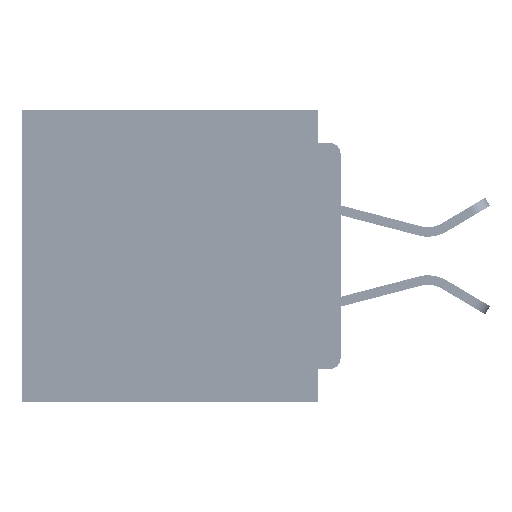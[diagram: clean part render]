
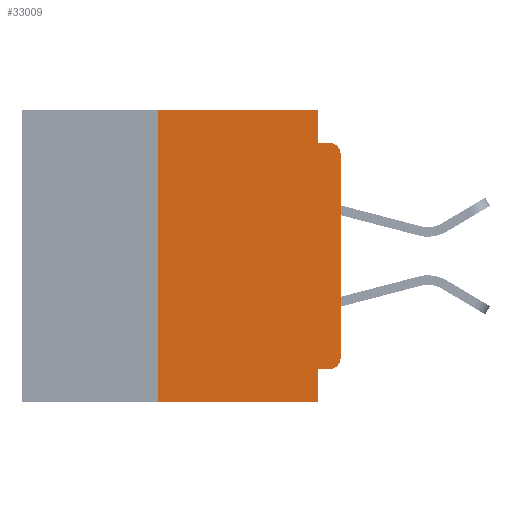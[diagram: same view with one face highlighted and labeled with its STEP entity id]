
A CAD part, left-side view. The second image highlights one B-rep face of the part: STEP entity #33009.
In plain terms, the highlighted planar face has unit normal (-1, 0, 0).
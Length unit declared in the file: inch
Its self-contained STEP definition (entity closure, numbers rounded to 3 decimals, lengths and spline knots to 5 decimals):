
#761 = CARTESIAN_POINT ( 'NONE',  ( 0., 0.031, -0.4 ) ) ;
#1078 = ORIENTED_EDGE ( 'NONE', *, *, #26324, .T. ) ;
#2343 = VECTOR ( 'NONE', #21626, 39.37008 ) ;
#2947 = AXIS2_PLACEMENT_3D ( 'NONE', #13943, #51163, #19364 ) ;
#2953 = DIRECTION ( 'NONE',  ( 0., 0., -1. ) ) ;
#3020 = VERTEX_POINT ( 'NONE', #41091 ) ;
#3185 = LINE ( 'NONE', #68620, #14150 ) ;
#3899 = VERTEX_POINT ( 'NONE', #10021 ) ;
#4468 = DIRECTION ( 'NONE',  ( 0., 0., 1. ) ) ;
#6984 = ORIENTED_EDGE ( 'NONE', *, *, #51844, .T. ) ;
#7105 = DIRECTION ( 'NONE',  ( 0., -1., 0. ) ) ;
#7507 = CARTESIAN_POINT ( 'NONE',  ( 0., 0.031, 0. ) ) ;
#8432 = CARTESIAN_POINT ( 'NONE',  ( 0., 0.437, -0.4 ) ) ;
#9477 = LINE ( 'NONE', #51518, #34702 ) ;
#10021 = CARTESIAN_POINT ( 'NONE',  ( 0., 0.015, -0.045 ) ) ;
#10410 = CIRCLE ( 'NONE', #2947, 0.015 ) ;
#11885 = CARTESIAN_POINT ( 'NONE',  ( 0., 0., -0.34 ) ) ;
#12005 = ORIENTED_EDGE ( 'NONE', *, *, #28152, .T. ) ;
#12892 = ORIENTED_EDGE ( 'NONE', *, *, #33095, .F. ) ;
#13035 = CARTESIAN_POINT ( 'NONE',  ( 0., 0.015, -0.34 ) ) ;
#13685 = VERTEX_POINT ( 'NONE', #55455 ) ;
#13847 = DIRECTION ( 'NONE',  ( 0., -1., 0. ) ) ;
#13943 = CARTESIAN_POINT ( 'NONE',  ( 0., 0.015, -0.06 ) ) ;
#14150 = VECTOR ( 'NONE', #31855, 39.37008 ) ;
#14158 = CARTESIAN_POINT ( 'NONE',  ( 0., 0.25, -0.4 ) ) ;
#15437 = VERTEX_POINT ( 'NONE', #17422 ) ;
#15997 = CARTESIAN_POINT ( 'NONE',  ( 0., 0.437, 0. ) ) ;
#16701 = LINE ( 'NONE', #15997, #2343 ) ;
#17422 = CARTESIAN_POINT ( 'NONE',  ( 0., 0., -0.06 ) ) ;
#18439 = DIRECTION ( 'NONE',  ( 0., 0., -1. ) ) ;
#19364 = DIRECTION ( 'NONE',  ( 0., 0., -1. ) ) ;
#21159 = VECTOR ( 'NONE', #13847, 39.37008 ) ;
#21319 = ORIENTED_EDGE ( 'NONE', *, *, #61310, .F. ) ;
#21379 = EDGE_CURVE ( 'NONE', #37187, #28528, #16701, .T. ) ;
#21626 = DIRECTION ( 'NONE',  ( 0., -1., 0. ) ) ;
#22849 = AXIS2_PLACEMENT_3D ( 'NONE', #66672, #35217, #2953 ) ;
#25450 = FACE_OUTER_BOUND ( 'NONE', #38545, .T. ) ;
#25771 = LINE ( 'NONE', #47013, #64611 ) ;
#26194 = VERTEX_POINT ( 'NONE', #761 ) ;
#26324 = EDGE_CURVE ( 'NONE', #13685, #67581, #44813, .T. ) ;
#27662 = CARTESIAN_POINT ( 'NONE',  ( 0., 0.031, -0.355 ) ) ;
#27998 = EDGE_CURVE ( 'NONE', #3020, #3899, #61105, .T. ) ;
#28152 = EDGE_CURVE ( 'NONE', #15437, #3899, #10410, .T. ) ;
#28528 = VERTEX_POINT ( 'NONE', #64459 ) ;
#30884 = CARTESIAN_POINT ( 'NONE',  ( 0., 0.25, 0. ) ) ;
#31855 = DIRECTION ( 'NONE',  ( 0., 0., -1. ) ) ;
#33009 = ADVANCED_FACE ( 'NONE', ( #25450 ), #61386, .F. ) ;
#33095 = EDGE_CURVE ( 'NONE', #51240, #37187, #9477, .T. ) ;
#34702 = VECTOR ( 'NONE', #46218, 39.37008 ) ;
#35217 = DIRECTION ( 'NONE',  ( 1., 0., 0. ) ) ;
#37187 = VERTEX_POINT ( 'NONE', #30884 ) ;
#38545 = EDGE_LOOP ( 'NONE', ( #38824, #12005, #54445, #61020, #39679, #12892, #6984, #21319, #68479, #1078 ) ) ;
#38752 = LINE ( 'NONE', #7507, #65068 ) ;
#38824 = ORIENTED_EDGE ( 'NONE', *, *, #62409, .T. ) ;
#39631 = DIRECTION ( 'NONE',  ( 0., 0., -1. ) ) ;
#39679 = ORIENTED_EDGE ( 'NONE', *, *, #21379, .F. ) ;
#41091 = CARTESIAN_POINT ( 'NONE',  ( 0., 0.031, -0.045 ) ) ;
#41942 = VECTOR ( 'NONE', #45950, 39.37008 ) ;
#44813 = CIRCLE ( 'NONE', #65723, 0.015 ) ;
#45950 = DIRECTION ( 'NONE',  ( 0., 1., 0. ) ) ;
#46218 = DIRECTION ( 'NONE',  ( 0., 0., 1. ) ) ;
#47013 = CARTESIAN_POINT ( 'NONE',  ( 0., 0., 0. ) ) ;
#47156 = VECTOR ( 'NONE', #7105, 39.37008 ) ;
#48330 = EDGE_CURVE ( 'NONE', #28528, #3020, #38752, .T. ) ;
#49097 = EDGE_CURVE ( 'NONE', #13685, #52197, #57541, .T. ) ;
#50265 = DIRECTION ( 'NONE',  ( -1., 0., 0. ) ) ;
#51163 = DIRECTION ( 'NONE',  ( -1., 0., 0. ) ) ;
#51240 = VERTEX_POINT ( 'NONE', #14158 ) ;
#51244 = CARTESIAN_POINT ( 'NONE',  ( 0., 0., -0.355 ) ) ;
#51518 = CARTESIAN_POINT ( 'NONE',  ( 0., 0.25, -0.4 ) ) ;
#51844 = EDGE_CURVE ( 'NONE', #51240, #26194, #63388, .T. ) ;
#52197 = VERTEX_POINT ( 'NONE', #27662 ) ;
#54445 = ORIENTED_EDGE ( 'NONE', *, *, #27998, .F. ) ;
#55455 = CARTESIAN_POINT ( 'NONE',  ( 0., 0.015, -0.355 ) ) ;
#57541 = LINE ( 'NONE', #51244, #41942 ) ;
#60132 = CARTESIAN_POINT ( 'NONE',  ( 0., 0., -0.045 ) ) ;
#61020 = ORIENTED_EDGE ( 'NONE', *, *, #48330, .F. ) ;
#61105 = LINE ( 'NONE', #60132, #47156 ) ;
#61310 = EDGE_CURVE ( 'NONE', #52197, #26194, #3185, .T. ) ;
#61386 = PLANE ( 'NONE',  #22849 ) ;
#62409 = EDGE_CURVE ( 'NONE', #67581, #15437, #25771, .T. ) ;
#63388 = LINE ( 'NONE', #8432, #21159 ) ;
#64459 = CARTESIAN_POINT ( 'NONE',  ( 0., 0.031, 0. ) ) ;
#64611 = VECTOR ( 'NONE', #4468, 39.37008 ) ;
#65068 = VECTOR ( 'NONE', #39631, 39.37008 ) ;
#65723 = AXIS2_PLACEMENT_3D ( 'NONE', #13035, #50265, #18439 ) ;
#66672 = CARTESIAN_POINT ( 'NONE',  ( 0., 0.437, 0. ) ) ;
#67581 = VERTEX_POINT ( 'NONE', #11885 ) ;
#68479 = ORIENTED_EDGE ( 'NONE', *, *, #49097, .F. ) ;
#68620 = CARTESIAN_POINT ( 'NONE',  ( 0., 0.031, -0.4 ) ) ;
